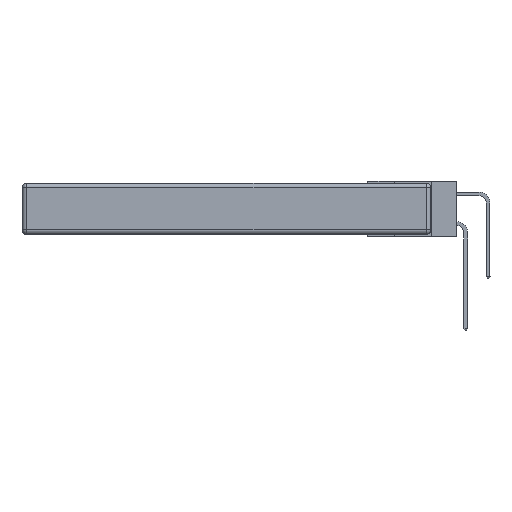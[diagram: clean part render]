
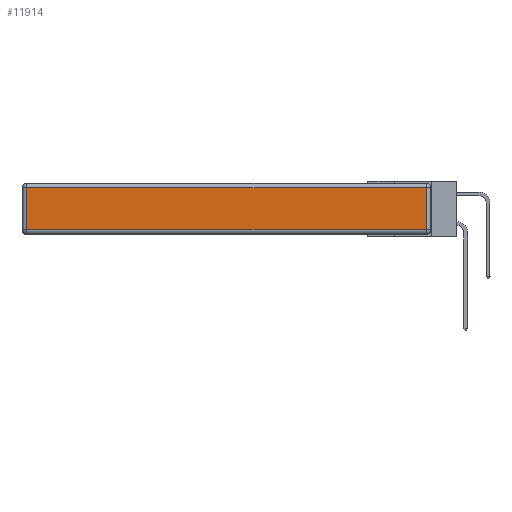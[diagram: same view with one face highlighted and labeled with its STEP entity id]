
A CAD part, left-side view. The second image highlights one B-rep face of the part: STEP entity #11914.
In plain terms, the highlighted planar face has unit normal (-1, 0, 0).
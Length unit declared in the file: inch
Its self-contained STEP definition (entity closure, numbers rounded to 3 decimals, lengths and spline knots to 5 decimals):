
#341 = FACE_OUTER_BOUND ( 'NONE', #782, .T. ) ;
#782 = EDGE_LOOP ( 'NONE', ( #13314, #1741, #11943, #5883 ) ) ;
#1006 = AXIS2_PLACEMENT_3D ( 'NONE', #21266, #12739, #8074 ) ;
#1741 = ORIENTED_EDGE ( 'NONE', *, *, #21108, .T. ) ;
#1998 = VERTEX_POINT ( 'NONE', #15791 ) ;
#2459 = VERTEX_POINT ( 'NONE', #25456 ) ;
#5682 = EDGE_CURVE ( 'NONE', #27269, #2459, #10190, .T. ) ;
#5883 = ORIENTED_EDGE ( 'NONE', *, *, #26125, .T. ) ;
#6329 = VECTOR ( 'NONE', #19159, 39.37008 ) ;
#8074 = DIRECTION ( 'NONE',  ( 0., 0., 1. ) ) ;
#8342 = EDGE_CURVE ( 'NONE', #1998, #15631, #15850, .T. ) ;
#9821 = DIRECTION ( 'NONE',  ( 0., 0., -1. ) ) ;
#10190 = LINE ( 'NONE', #11912, #19386 ) ;
#11819 = DIRECTION ( 'NONE',  ( 0., 0., 1. ) ) ;
#11912 = CARTESIAN_POINT ( 'NONE',  ( 0., 2.75, -0.03 ) ) ;
#11914 = ADVANCED_FACE ( 'NONE', ( #341 ), #21082, .T. ) ;
#11943 = ORIENTED_EDGE ( 'NONE', *, *, #5682, .T. ) ;
#12739 = DIRECTION ( 'NONE',  ( -1., 0., 0. ) ) ;
#12997 = CARTESIAN_POINT ( 'NONE',  ( 0., 0., -0.313 ) ) ;
#13314 = ORIENTED_EDGE ( 'NONE', *, *, #8342, .T. ) ;
#14854 = VECTOR ( 'NONE', #9821, 39.37008 ) ;
#15631 = VERTEX_POINT ( 'NONE', #20445 ) ;
#15791 = CARTESIAN_POINT ( 'NONE',  ( 0., 2.72, -0.313 ) ) ;
#15850 = LINE ( 'NONE', #12997, #6329 ) ;
#15925 = CARTESIAN_POINT ( 'NONE',  ( 0., 0.03, -0.343 ) ) ;
#17091 = CARTESIAN_POINT ( 'NONE',  ( 0., 0.03, -0.03 ) ) ;
#18381 = DIRECTION ( 'NONE',  ( 0., 1., 0. ) ) ;
#18907 = VECTOR ( 'NONE', #11819, 39.37008 ) ;
#19159 = DIRECTION ( 'NONE',  ( 0., -1., 0. ) ) ;
#19386 = VECTOR ( 'NONE', #18381, 39.37008 ) ;
#20445 = CARTESIAN_POINT ( 'NONE',  ( 0., 0.03, -0.313 ) ) ;
#21082 = PLANE ( 'NONE',  #1006 ) ;
#21108 = EDGE_CURVE ( 'NONE', #15631, #27269, #24713, .T. ) ;
#21266 = CARTESIAN_POINT ( 'NONE',  ( 0., 0., -0.343 ) ) ;
#21312 = LINE ( 'NONE', #22656, #14854 ) ;
#22656 = CARTESIAN_POINT ( 'NONE',  ( 0., 2.72, -0.343 ) ) ;
#24713 = LINE ( 'NONE', #15925, #18907 ) ;
#25456 = CARTESIAN_POINT ( 'NONE',  ( 0., 2.72, -0.03 ) ) ;
#26125 = EDGE_CURVE ( 'NONE', #2459, #1998, #21312, .T. ) ;
#27269 = VERTEX_POINT ( 'NONE', #17091 ) ;
